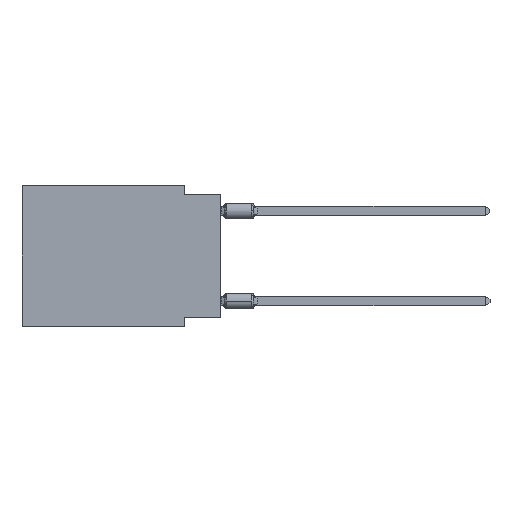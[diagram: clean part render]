
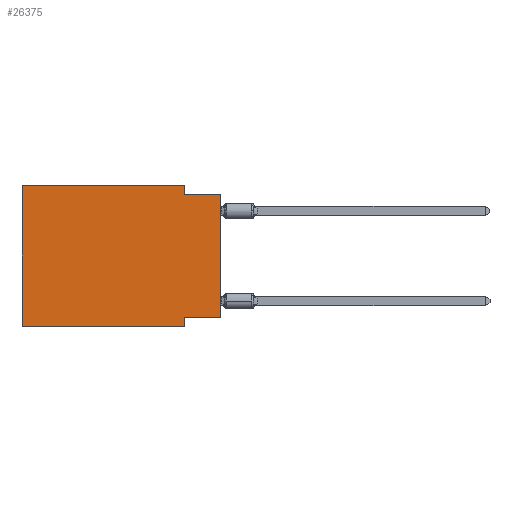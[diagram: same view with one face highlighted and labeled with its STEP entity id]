
A CAD part, left-side view. The second image highlights one B-rep face of the part: STEP entity #26375.
In plain terms, the highlighted planar face has unit normal (-1, 0, 0).
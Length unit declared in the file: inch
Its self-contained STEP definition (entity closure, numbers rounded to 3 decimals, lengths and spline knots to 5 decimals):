
#1152 = DIRECTION ( 'NONE',  ( 0., 0., 1. ) ) ;
#1510 = CARTESIAN_POINT ( 'NONE',  ( 0., 0.55, 0. ) ) ;
#1915 = DIRECTION ( 'NONE',  ( 0., 1., 0. ) ) ;
#2031 = DIRECTION ( 'NONE',  ( 0., 0., -1. ) ) ;
#2961 = LINE ( 'NONE', #10644, #8899 ) ;
#6737 = VERTEX_POINT ( 'NONE', #15936 ) ;
#7344 = AXIS2_PLACEMENT_3D ( 'NONE', #20041, #19252, #47542 ) ;
#7686 = CARTESIAN_POINT ( 'NONE',  ( 0., 0.1, -0.365 ) ) ;
#8459 = VERTEX_POINT ( 'NONE', #7686 ) ;
#8899 = VECTOR ( 'NONE', #23300, 39.37008 ) ;
#9351 = LINE ( 'NONE', #29701, #28787 ) ;
#10450 = VECTOR ( 'NONE', #26907, 39.37008 ) ;
#10644 = CARTESIAN_POINT ( 'NONE',  ( 0., 0., -0.025 ) ) ;
#10976 = DIRECTION ( 'NONE',  ( 0., -1., 0. ) ) ;
#11473 = VECTOR ( 'NONE', #10976, 39.37008 ) ;
#13287 = EDGE_LOOP ( 'NONE', ( #35800, #24889, #40038, #22426, #33014, #50360, #35078, #36016 ) ) ;
#13598 = VECTOR ( 'NONE', #30447, 39.37008 ) ;
#15936 = CARTESIAN_POINT ( 'NONE',  ( 0., 0., -0.365 ) ) ;
#16089 = CARTESIAN_POINT ( 'NONE',  ( 0., 0., -0.025 ) ) ;
#16315 = EDGE_CURVE ( 'NONE', #6737, #8459, #9351, .T. ) ;
#18180 = CARTESIAN_POINT ( 'NONE',  ( 0., 0.55, 0. ) ) ;
#18577 = VERTEX_POINT ( 'NONE', #41306 ) ;
#18709 = LINE ( 'NONE', #18180, #31447 ) ;
#18764 = CARTESIAN_POINT ( 'NONE',  ( 0., 0.1, -0.025 ) ) ;
#18916 = VERTEX_POINT ( 'NONE', #18764 ) ;
#19252 = DIRECTION ( 'NONE',  ( 1., 0., 0. ) ) ;
#19279 = EDGE_CURVE ( 'NONE', #6737, #40659, #50928, .T. ) ;
#20041 = CARTESIAN_POINT ( 'NONE',  ( 0., 0.55, 0. ) ) ;
#20963 = CARTESIAN_POINT ( 'NONE',  ( 0., 0.55, 0. ) ) ;
#21753 = VERTEX_POINT ( 'NONE', #49989 ) ;
#22426 = ORIENTED_EDGE ( 'NONE', *, *, #48398, .F. ) ;
#23136 = EDGE_CURVE ( 'NONE', #18577, #24001, #51905, .T. ) ;
#23300 = DIRECTION ( 'NONE',  ( 0., -1., 0. ) ) ;
#24001 = VERTEX_POINT ( 'NONE', #28810 ) ;
#24889 = ORIENTED_EDGE ( 'NONE', *, *, #32977, .F. ) ;
#25706 = CARTESIAN_POINT ( 'NONE',  ( 0., 0.1, 0. ) ) ;
#26375 = ADVANCED_FACE ( 'NONE', ( #28250 ), #52009, .F. ) ;
#26907 = DIRECTION ( 'NONE',  ( 0., 0., 1. ) ) ;
#26918 = DIRECTION ( 'NONE',  ( 0., -1., 0. ) ) ;
#27887 = CARTESIAN_POINT ( 'NONE',  ( 0., 0.55, -0.39 ) ) ;
#28250 = FACE_OUTER_BOUND ( 'NONE', #13287, .T. ) ;
#28787 = VECTOR ( 'NONE', #1915, 39.37008 ) ;
#28810 = CARTESIAN_POINT ( 'NONE',  ( 0., 0.1, -0.39 ) ) ;
#29697 = LINE ( 'NONE', #25706, #13598 ) ;
#29701 = CARTESIAN_POINT ( 'NONE',  ( 0., 0., -0.365 ) ) ;
#30447 = DIRECTION ( 'NONE',  ( 0., 0., -1. ) ) ;
#30869 = CARTESIAN_POINT ( 'NONE',  ( 0., 0., 0. ) ) ;
#31447 = VECTOR ( 'NONE', #26918, 39.37008 ) ;
#32977 = EDGE_CURVE ( 'NONE', #18916, #40659, #2961, .T. ) ;
#33014 = ORIENTED_EDGE ( 'NONE', *, *, #37275, .F. ) ;
#35078 = ORIENTED_EDGE ( 'NONE', *, *, #43710, .F. ) ;
#35800 = ORIENTED_EDGE ( 'NONE', *, *, #19279, .T. ) ;
#36016 = ORIENTED_EDGE ( 'NONE', *, *, #16315, .F. ) ;
#36967 = VECTOR ( 'NONE', #1152, 39.37008 ) ;
#37275 = EDGE_CURVE ( 'NONE', #18577, #47550, #37876, .T. ) ;
#37876 = LINE ( 'NONE', #20963, #36967 ) ;
#38241 = CARTESIAN_POINT ( 'NONE',  ( 0., 0.1, -0.39 ) ) ;
#38499 = LINE ( 'NONE', #38241, #49090 ) ;
#40038 = ORIENTED_EDGE ( 'NONE', *, *, #41619, .F. ) ;
#40659 = VERTEX_POINT ( 'NONE', #16089 ) ;
#41306 = CARTESIAN_POINT ( 'NONE',  ( 0., 0.55, -0.39 ) ) ;
#41619 = EDGE_CURVE ( 'NONE', #21753, #18916, #29697, .T. ) ;
#43710 = EDGE_CURVE ( 'NONE', #8459, #24001, #38499, .T. ) ;
#47542 = DIRECTION ( 'NONE',  ( 0., 0., -1. ) ) ;
#47550 = VERTEX_POINT ( 'NONE', #1510 ) ;
#48398 = EDGE_CURVE ( 'NONE', #47550, #21753, #18709, .T. ) ;
#49090 = VECTOR ( 'NONE', #2031, 39.37008 ) ;
#49989 = CARTESIAN_POINT ( 'NONE',  ( 0., 0.1, 0. ) ) ;
#50360 = ORIENTED_EDGE ( 'NONE', *, *, #23136, .T. ) ;
#50928 = LINE ( 'NONE', #30869, #10450 ) ;
#51905 = LINE ( 'NONE', #27887, #11473 ) ;
#52009 = PLANE ( 'NONE',  #7344 ) ;
